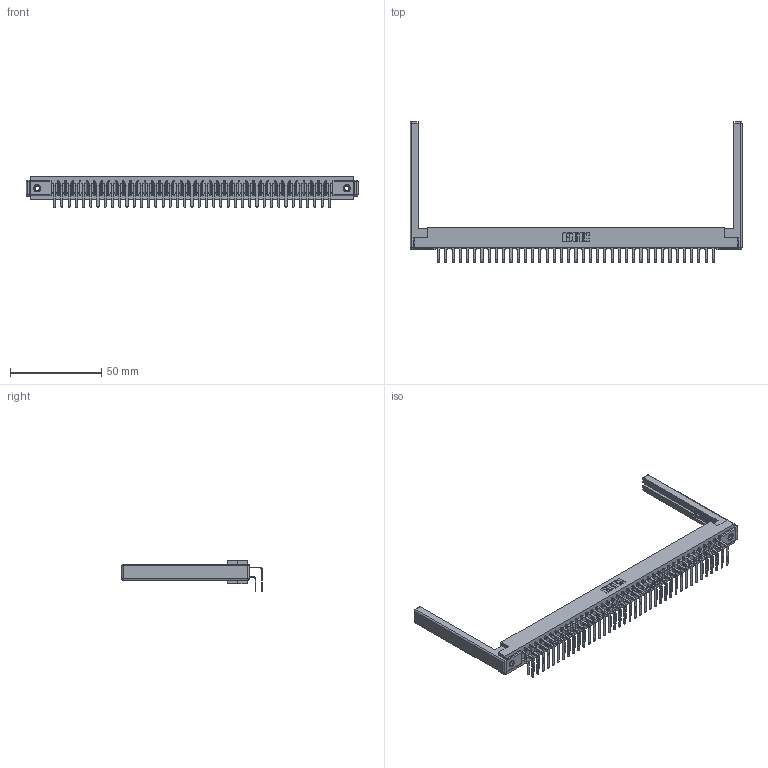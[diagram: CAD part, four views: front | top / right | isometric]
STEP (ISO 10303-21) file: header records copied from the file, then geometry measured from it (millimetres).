
FILE_DESCRIPTION (( 'STEP AP203' ), '1' );
FILE_NAME ('307-078-558-268.STEP', '2019-09-06T23:15:22', ( '' ), ( '' ), 'SwSTEP 2.0', 'SolidWorks 2016', '' );
FILE_SCHEMA (( 'CONFIG_CONTROL_DESIGN' ));
Length unit declared in the file: inch
Products named in the file (6): 307 Part_.156 Dia Mounting Holes; 307-220-068; 307-078-558-268; 307-290-001_558 559 - 1 (Single); 345-250-001_345-250-001-102; 307-290-001_558 - 2 (Single)
Assembly tree (83 placements, depth 2):
  307-078-558-268
    307 Part_.156 Dia Mounting Holes
    307-290-001_558 559 - 1 (Single)  x39
    307-290-001_558 - 2 (Single)  x39
    307-220-068  x2
    345-250-001_345-250-001-102  x2
Bounding box: 181.97 x 76.92 x 16.8 mm (x, y, z)
Volume: 24055 mm3; surface area: 30008.7 mm2
Topology: 83 solids, 83 shells, 4212 faces, 11789 edges, 7626 vertices
Faces by surface type: plane 2732, cylinder 1376, sphere 88, cone 12, torus 4
Entity records: 39258 total; most frequent: CARTESIAN_POINT 6402, ORIENTED_EDGE 6336, DIRECTION 6286, EDGE_CURVE 3168, VECTOR 2426, LINE 2426, VERTEX_POINT 2046, AXIS2_PLACEMENT_3D 1930
